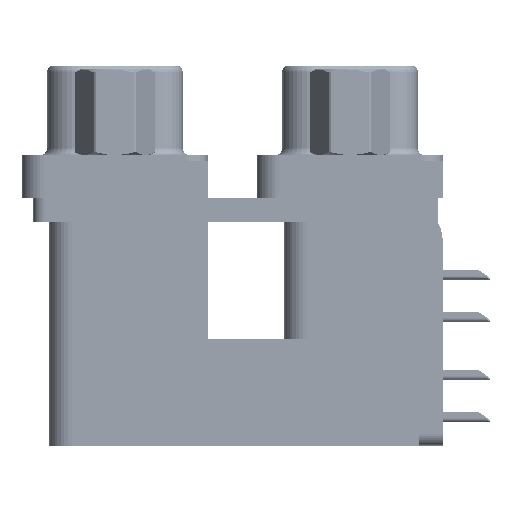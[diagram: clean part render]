
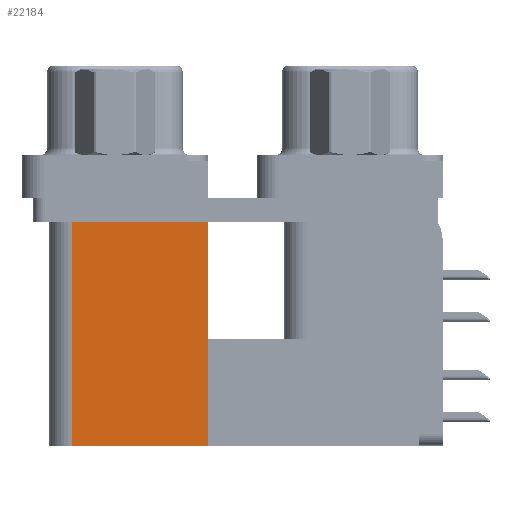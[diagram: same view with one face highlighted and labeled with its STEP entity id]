
A CAD part, left-side view. The second image highlights one B-rep face of the part: STEP entity #22184.
In plain terms, the highlighted planar face has unit normal (-1, 0, 0).
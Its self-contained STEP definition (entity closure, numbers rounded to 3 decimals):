
#1363 = VERTEX_POINT ( 'NONE', #3349 ) ;
#2423 = CARTESIAN_POINT ( 'NONE',  ( 3.79, 9.6, -19.2 ) ) ;
#3349 = CARTESIAN_POINT ( 'NONE',  ( 3.79, 9.6, -2.5 ) ) ;
#3531 = VECTOR ( 'NONE', #29209, 1000. ) ;
#5643 = VERTEX_POINT ( 'NONE', #15959 ) ;
#6213 = ORIENTED_EDGE ( 'NONE', *, *, #17021, .T. ) ;
#6947 = LINE ( 'NONE', #28082, #16365 ) ;
#7720 = DIRECTION ( 'NONE',  ( 0., 1., 0. ) ) ;
#8393 = FACE_OUTER_BOUND ( 'NONE', #20349, .T. ) ;
#9302 = VECTOR ( 'NONE', #17141, 1000. ) ;
#10078 = ORIENTED_EDGE ( 'NONE', *, *, #52600, .F. ) ;
#11398 = CARTESIAN_POINT ( 'NONE',  ( 3.79, 9.6, -2.5 ) ) ;
#12919 = LINE ( 'NONE', #15531, #9302 ) ;
#15531 = CARTESIAN_POINT ( 'NONE',  ( 3.79, 18.8, -19.2 ) ) ;
#15623 = LINE ( 'NONE', #11398, #16971 ) ;
#15959 = CARTESIAN_POINT ( 'NONE',  ( 3.79, 18.8, -19.2 ) ) ;
#16365 = VECTOR ( 'NONE', #19359, 1000. ) ;
#16971 = VECTOR ( 'NONE', #7720, 1000. ) ;
#17021 = EDGE_CURVE ( 'NONE', #29277, #1363, #32864, .T. ) ;
#17141 = DIRECTION ( 'NONE',  ( 0., 0., 1. ) ) ;
#17419 = PLANE ( 'NONE',  #23222 ) ;
#19359 = DIRECTION ( 'NONE',  ( 0., 1., 0. ) ) ;
#20349 = EDGE_LOOP ( 'NONE', ( #40218, #46255, #10078, #6213 ) ) ;
#22184 = ADVANCED_FACE ( 'NONE', ( #8393 ), #17419, .F. ) ;
#22534 = EDGE_CURVE ( 'NONE', #1363, #33277, #15623, .T. ) ;
#23222 = AXIS2_PLACEMENT_3D ( 'NONE', #47251, #37710, #43030 ) ;
#24457 = CARTESIAN_POINT ( 'NONE',  ( 3.79, 9.6, -19.2 ) ) ;
#28082 = CARTESIAN_POINT ( 'NONE',  ( 3.79, 9.6, -19.2 ) ) ;
#29209 = DIRECTION ( 'NONE',  ( 0., 0., 1. ) ) ;
#29277 = VERTEX_POINT ( 'NONE', #2423 ) ;
#31475 = CARTESIAN_POINT ( 'NONE',  ( 3.79, 18.8, -2.5 ) ) ;
#32864 = LINE ( 'NONE', #24457, #3531 ) ;
#33277 = VERTEX_POINT ( 'NONE', #31475 ) ;
#37710 = DIRECTION ( 'NONE',  ( 1., 0., 0. ) ) ;
#40218 = ORIENTED_EDGE ( 'NONE', *, *, #22534, .T. ) ;
#43030 = DIRECTION ( 'NONE',  ( 0., 0., -1. ) ) ;
#46255 = ORIENTED_EDGE ( 'NONE', *, *, #54936, .F. ) ;
#47251 = CARTESIAN_POINT ( 'NONE',  ( 3.79, 9.6, -19.2 ) ) ;
#52600 = EDGE_CURVE ( 'NONE', #29277, #5643, #6947, .T. ) ;
#54936 = EDGE_CURVE ( 'NONE', #5643, #33277, #12919, .T. ) ;
